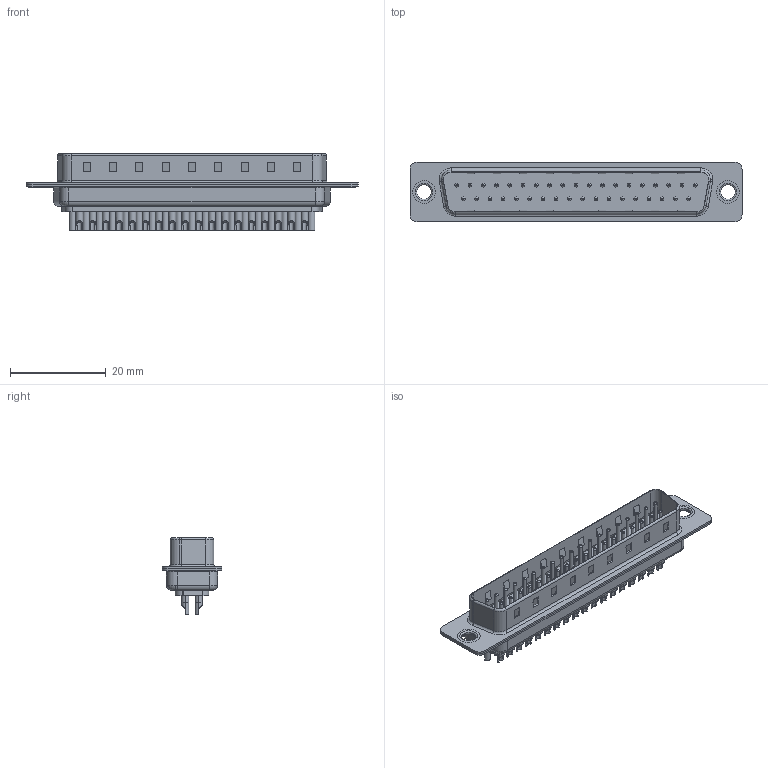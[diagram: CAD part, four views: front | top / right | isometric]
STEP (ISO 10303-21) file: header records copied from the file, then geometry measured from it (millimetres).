
FILE_DESCRIPTION (( 'STEP AP203' ), '1' );
FILE_NAME ('627-M37-622-WN1.STEP', '2021-04-23T15:55:54', ( '' ), ( '' ), 'SwSTEP 2.0', 'SolidWorks 2020', '' );
FILE_SCHEMA (( 'CONFIG_CONTROL_DESIGN' ));
Length unit declared in the file: millimetre
Products named in the file (7): 627-M37-622-WN1; 627M Shell Rear_37 Contacts; 627M Contact Row 2_22; 627M Shell Front_37 Contacts; 627M Contact Row 1_22; 627M Housing_37 Contacts; 627M Thru Hole Rivet
Assembly tree (42 placements, depth 2):
  627-M37-622-WN1
    627M Housing_37 Contacts
    627M Shell Front_37 Contacts
    627M Shell Rear_37 Contacts
    627M Contact Row 1_22  x19
    627M Contact Row 2_22  x18
    627M Thru Hole Rivet  x2
Bounding box: 69.4 x 12.5 x 16.05 mm (x, y, z)
Volume: 3774.4 mm3; surface area: 9470.9 mm2
Topology: 42 solids, 42 shells, 1755 faces, 4083 edges, 2497 vertices
Faces by surface type: cylinder 717, plane 536, torus 428, cone 74
Entity records: 23297 total; most frequent: DIRECTION 4037, CARTESIAN_POINT 3738, ORIENTED_EDGE 3458, EDGE_CURVE 1729, AXIS2_PLACEMENT_3D 1578, VERTEX_POINT 1108, EDGE_LOOP 931, VECTOR 881
